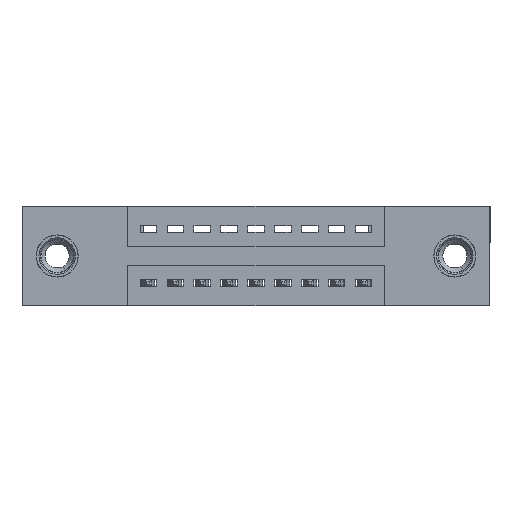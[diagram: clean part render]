
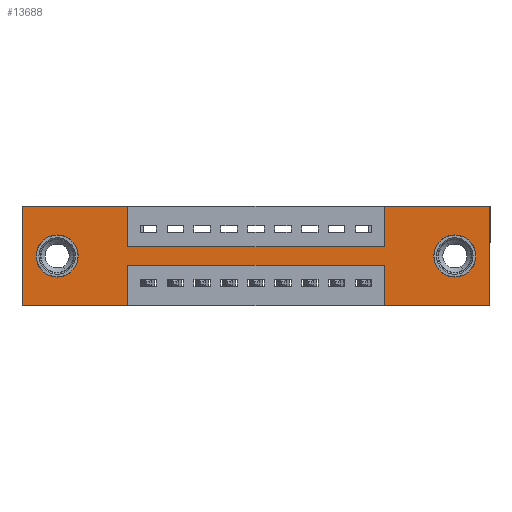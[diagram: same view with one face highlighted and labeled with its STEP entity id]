
A CAD part, front view. The second image highlights one B-rep face of the part: STEP entity #13688.
In plain terms, the highlighted planar face has unit normal (0, -1, 0).
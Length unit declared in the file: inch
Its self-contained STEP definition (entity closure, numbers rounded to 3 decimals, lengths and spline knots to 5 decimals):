
#1 = CARTESIAN_POINT ( 'NONE',  ( 0., 0., 0. ) ) ;
#94 = CARTESIAN_POINT ( 'NONE',  ( 0., 0., -0.37 ) ) ;
#120 = ORIENTED_EDGE ( 'NONE', *, *, #14578, .F. ) ;
#194 = VECTOR ( 'NONE', #6779, 39.37008 ) ;
#228 = DIRECTION ( 'NONE',  ( 1., 0., 0. ) ) ;
#270 = VERTEX_POINT ( 'NONE', #10863 ) ;
#312 = FACE_BOUND ( 'NONE', #3456, .T. ) ;
#343 = DIRECTION ( 'NONE',  ( 0., 1., 0. ) ) ;
#389 = EDGE_CURVE ( 'NONE', #10277, #10554, #5670, .T. ) ;
#649 = CARTESIAN_POINT ( 'NONE',  ( 0., 0., -0.37 ) ) ;
#875 = CARTESIAN_POINT ( 'NONE',  ( 0.3925, 0., -0.22 ) ) ;
#895 = AXIS2_PLACEMENT_3D ( 'NONE', #7783, #343, #8916 ) ;
#1064 = EDGE_LOOP ( 'NONE', ( #11375, #7035 ) ) ;
#1290 = PLANE ( 'NONE',  #2909 ) ;
#1365 = CARTESIAN_POINT ( 'NONE',  ( 0.13, 0., -0.185 ) ) ;
#1507 = DIRECTION ( 'NONE',  ( -1., 0., 0. ) ) ;
#1523 = EDGE_CURVE ( 'NONE', #270, #9955, #14107, .T. ) ;
#1527 = VERTEX_POINT ( 'NONE', #10328 ) ;
#1659 = LINE ( 'NONE', #5903, #4951 ) ;
#1786 = ORIENTED_EDGE ( 'NONE', *, *, #10797, .F. ) ;
#2102 = EDGE_CURVE ( 'NONE', #10007, #10277, #7556, .T. ) ;
#2225 = CARTESIAN_POINT ( 'NONE',  ( 0.3925, 0., -0.15 ) ) ;
#2279 = ORIENTED_EDGE ( 'NONE', *, *, #3471, .F. ) ;
#2285 = VERTEX_POINT ( 'NONE', #9213 ) ;
#2362 = CARTESIAN_POINT ( 'NONE',  ( 1.3425, 0., 0. ) ) ;
#2454 = CARTESIAN_POINT ( 'NONE',  ( 0.13, 0., -0.185 ) ) ;
#2516 = VERTEX_POINT ( 'NONE', #15848 ) ;
#2624 = CARTESIAN_POINT ( 'NONE',  ( 1.605, 0., -0.185 ) ) ;
#2644 = ORIENTED_EDGE ( 'NONE', *, *, #2102, .F. ) ;
#2909 = AXIS2_PLACEMENT_3D ( 'NONE', #94, #5026, #4912 ) ;
#3162 = CARTESIAN_POINT ( 'NONE',  ( 0.3925, 0., 0. ) ) ;
#3431 = DIRECTION ( 'NONE',  ( 1., 0., 0. ) ) ;
#3456 = EDGE_LOOP ( 'NONE', ( #8382, #13320 ) ) ;
#3471 = EDGE_CURVE ( 'NONE', #5555, #6298, #15402, .T. ) ;
#3636 = AXIS2_PLACEMENT_3D ( 'NONE', #2624, #3812, #9893 ) ;
#3696 = DIRECTION ( 'NONE',  ( 0., 0., 1. ) ) ;
#3812 = DIRECTION ( 'NONE',  ( 0., 1., 0. ) ) ;
#3878 = EDGE_LOOP ( 'NONE', ( #14241, #2279, #1786, #4183, #10481, #9183, #11618, #5689, #120, #7195, #11658, #2644 ) ) ;
#4183 = ORIENTED_EDGE ( 'NONE', *, *, #9384, .F. ) ;
#4186 = FACE_OUTER_BOUND ( 'NONE', #3878, .T. ) ;
#4348 = VECTOR ( 'NONE', #11640, 39.37008 ) ;
#4392 = VERTEX_POINT ( 'NONE', #10001 ) ;
#4441 = EDGE_CURVE ( 'NONE', #12866, #4392, #5746, .T. ) ;
#4720 = CARTESIAN_POINT ( 'NONE',  ( 0., 0., 0. ) ) ;
#4912 = DIRECTION ( 'NONE',  ( 0., 0., -1. ) ) ;
#4951 = VECTOR ( 'NONE', #8289, 39.37008 ) ;
#4964 = FACE_BOUND ( 'NONE', #1064, .T. ) ;
#5026 = DIRECTION ( 'NONE',  ( 0., -1., 0. ) ) ;
#5077 = AXIS2_PLACEMENT_3D ( 'NONE', #1365, #12892, #9153 ) ;
#5094 = VERTEX_POINT ( 'NONE', #13680 ) ;
#5555 = VERTEX_POINT ( 'NONE', #5666 ) ;
#5666 = CARTESIAN_POINT ( 'NONE',  ( 1.3425, 0., -0.22 ) ) ;
#5670 = LINE ( 'NONE', #4720, #10681 ) ;
#5676 = VERTEX_POINT ( 'NONE', #7243 ) ;
#5689 = ORIENTED_EDGE ( 'NONE', *, *, #4441, .F. ) ;
#5746 = LINE ( 'NONE', #2225, #10355 ) ;
#5903 = CARTESIAN_POINT ( 'NONE',  ( 1.735, 0., 0. ) ) ;
#5912 = CARTESIAN_POINT ( 'NONE',  ( 0., 0., 0. ) ) ;
#5941 = EDGE_CURVE ( 'NONE', #13030, #14690, #6450, .T. ) ;
#6298 = VERTEX_POINT ( 'NONE', #10198 ) ;
#6420 = CARTESIAN_POINT ( 'NONE',  ( 0., 0., -0.37 ) ) ;
#6450 = LINE ( 'NONE', #5912, #11615 ) ;
#6779 = DIRECTION ( 'NONE',  ( -1., 0., 0. ) ) ;
#7035 = ORIENTED_EDGE ( 'NONE', *, *, #1523, .T. ) ;
#7195 = ORIENTED_EDGE ( 'NONE', *, *, #13007, .F. ) ;
#7243 = CARTESIAN_POINT ( 'NONE',  ( 0.13, 0., -0.263 ) ) ;
#7318 = VECTOR ( 'NONE', #12107, 39.37008 ) ;
#7556 = LINE ( 'NONE', #6420, #194 ) ;
#7638 = LINE ( 'NONE', #3162, #4348 ) ;
#7754 = CARTESIAN_POINT ( 'NONE',  ( 1.3425, 0., -0.37 ) ) ;
#7783 = CARTESIAN_POINT ( 'NONE',  ( 1.605, 0., -0.185 ) ) ;
#7864 = CIRCLE ( 'NONE', #3636, 0.078 ) ;
#7926 = CARTESIAN_POINT ( 'NONE',  ( 0.3925, 0., -0.37 ) ) ;
#8289 = DIRECTION ( 'NONE',  ( 0., 0., -1. ) ) ;
#8382 = ORIENTED_EDGE ( 'NONE', *, *, #14982, .T. ) ;
#8431 = DIRECTION ( 'NONE',  ( 0., 0., 1. ) ) ;
#8598 = DIRECTION ( 'NONE',  ( 0., 0., 1. ) ) ;
#8730 = EDGE_CURVE ( 'NONE', #4392, #13030, #11817, .T. ) ;
#8907 = CARTESIAN_POINT ( 'NONE',  ( 0., 0., 0. ) ) ;
#8916 = DIRECTION ( 'NONE',  ( 0., 0., -1. ) ) ;
#8993 = DIRECTION ( 'NONE',  ( 0., 0., 1. ) ) ;
#9086 = LINE ( 'NONE', #7926, #11403 ) ;
#9153 = DIRECTION ( 'NONE',  ( 0., 0., 1. ) ) ;
#9183 = ORIENTED_EDGE ( 'NONE', *, *, #5941, .F. ) ;
#9213 = CARTESIAN_POINT ( 'NONE',  ( 1.735, 0., -0.37 ) ) ;
#9384 = EDGE_CURVE ( 'NONE', #2285, #5094, #15880, .T. ) ;
#9893 = DIRECTION ( 'NONE',  ( 0., 0., -1. ) ) ;
#9955 = VERTEX_POINT ( 'NONE', #13790 ) ;
#10001 = CARTESIAN_POINT ( 'NONE',  ( 1.3425, 0., -0.15 ) ) ;
#10007 = VERTEX_POINT ( 'NONE', #15353 ) ;
#10198 = CARTESIAN_POINT ( 'NONE',  ( 0.3925, 0., -0.22 ) ) ;
#10277 = VERTEX_POINT ( 'NONE', #649 ) ;
#10320 = EDGE_CURVE ( 'NONE', #6298, #10007, #9086, .T. ) ;
#10328 = CARTESIAN_POINT ( 'NONE',  ( 0.3925, 0., 0. ) ) ;
#10355 = VECTOR ( 'NONE', #14887, 39.37008 ) ;
#10426 = AXIS2_PLACEMENT_3D ( 'NONE', #2454, #11063, #3696 ) ;
#10481 = ORIENTED_EDGE ( 'NONE', *, *, #15376, .F. ) ;
#10554 = VERTEX_POINT ( 'NONE', #1 ) ;
#10619 = LINE ( 'NONE', #7754, #15451 ) ;
#10681 = VECTOR ( 'NONE', #8598, 39.37008 ) ;
#10797 = EDGE_CURVE ( 'NONE', #5094, #5555, #10619, .T. ) ;
#10811 = CARTESIAN_POINT ( 'NONE',  ( 1.735, 0., 0. ) ) ;
#10863 = CARTESIAN_POINT ( 'NONE',  ( 1.605, 0., -0.263 ) ) ;
#11063 = DIRECTION ( 'NONE',  ( 0., 1., 0. ) ) ;
#11375 = ORIENTED_EDGE ( 'NONE', *, *, #12291, .T. ) ;
#11403 = VECTOR ( 'NONE', #11630, 39.37008 ) ;
#11615 = VECTOR ( 'NONE', #3431, 39.37008 ) ;
#11618 = ORIENTED_EDGE ( 'NONE', *, *, #8730, .F. ) ;
#11630 = DIRECTION ( 'NONE',  ( 0., 0., -1. ) ) ;
#11640 = DIRECTION ( 'NONE',  ( 0., 0., -1. ) ) ;
#11658 = ORIENTED_EDGE ( 'NONE', *, *, #389, .F. ) ;
#11817 = LINE ( 'NONE', #2362, #13393 ) ;
#12107 = DIRECTION ( 'NONE',  ( -1., 0., 0. ) ) ;
#12259 = CIRCLE ( 'NONE', #5077, 0.078 ) ;
#12291 = EDGE_CURVE ( 'NONE', #9955, #270, #7864, .T. ) ;
#12297 = LINE ( 'NONE', #8907, #13044 ) ;
#12418 = VECTOR ( 'NONE', #1507, 39.37008 ) ;
#12866 = VERTEX_POINT ( 'NONE', #15906 ) ;
#12892 = DIRECTION ( 'NONE',  ( 0., 1., 0. ) ) ;
#13007 = EDGE_CURVE ( 'NONE', #10554, #1527, #12297, .T. ) ;
#13030 = VERTEX_POINT ( 'NONE', #14807 ) ;
#13044 = VECTOR ( 'NONE', #228, 39.37008 ) ;
#13320 = ORIENTED_EDGE ( 'NONE', *, *, #13657, .T. ) ;
#13393 = VECTOR ( 'NONE', #8431, 39.37008 ) ;
#13657 = EDGE_CURVE ( 'NONE', #5676, #2516, #14210, .T. ) ;
#13680 = CARTESIAN_POINT ( 'NONE',  ( 1.3425, 0., -0.37 ) ) ;
#13688 = ADVANCED_FACE ( 'NONE', ( #4964, #312, #4186 ), #1290, .T. ) ;
#13790 = CARTESIAN_POINT ( 'NONE',  ( 1.605, 0., -0.107 ) ) ;
#14107 = CIRCLE ( 'NONE', #895, 0.078 ) ;
#14210 = CIRCLE ( 'NONE', #10426, 0.078 ) ;
#14241 = ORIENTED_EDGE ( 'NONE', *, *, #10320, .F. ) ;
#14578 = EDGE_CURVE ( 'NONE', #1527, #12866, #7638, .T. ) ;
#14690 = VERTEX_POINT ( 'NONE', #10811 ) ;
#14807 = CARTESIAN_POINT ( 'NONE',  ( 1.3425, 0., 0. ) ) ;
#14887 = DIRECTION ( 'NONE',  ( 1., 0., 0. ) ) ;
#14948 = CARTESIAN_POINT ( 'NONE',  ( 0., 0., -0.37 ) ) ;
#14982 = EDGE_CURVE ( 'NONE', #2516, #5676, #12259, .T. ) ;
#15353 = CARTESIAN_POINT ( 'NONE',  ( 0.3925, 0., -0.37 ) ) ;
#15376 = EDGE_CURVE ( 'NONE', #14690, #2285, #1659, .T. ) ;
#15402 = LINE ( 'NONE', #875, #7318 ) ;
#15451 = VECTOR ( 'NONE', #8993, 39.37008 ) ;
#15848 = CARTESIAN_POINT ( 'NONE',  ( 0.13, 0., -0.107 ) ) ;
#15880 = LINE ( 'NONE', #14948, #12418 ) ;
#15906 = CARTESIAN_POINT ( 'NONE',  ( 0.3925, 0., -0.15 ) ) ;
